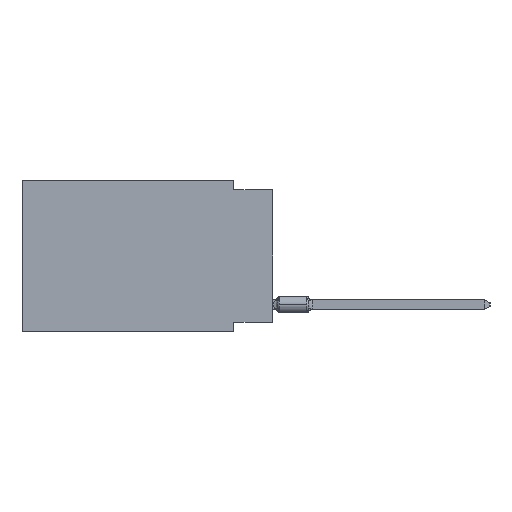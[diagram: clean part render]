
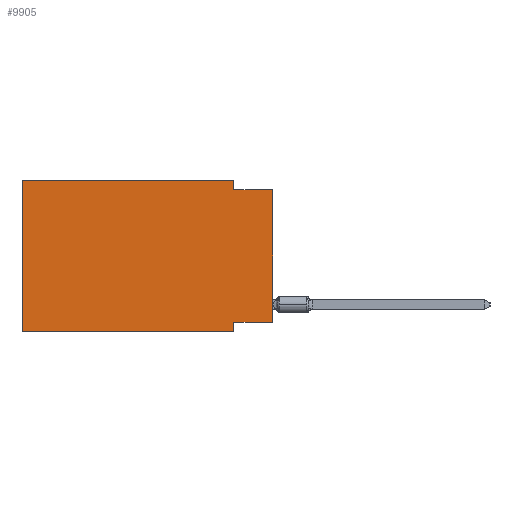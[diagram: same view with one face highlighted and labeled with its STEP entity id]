
A CAD part, left-side view. The second image highlights one B-rep face of the part: STEP entity #9905.
In plain terms, the highlighted planar face has unit normal (-1, 0, 0).
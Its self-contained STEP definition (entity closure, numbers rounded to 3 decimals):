
#143 = CARTESIAN_POINT ( 'NONE',  ( 0., 2.54, 0. ) ) ;
#326 = VERTEX_POINT ( 'NONE', #11461 ) ;
#494 = FACE_OUTER_BOUND ( 'NONE', #1102, .T. ) ;
#961 = CARTESIAN_POINT ( 'NONE',  ( 0., 0., -0.635 ) ) ;
#1102 = EDGE_LOOP ( 'NONE', ( #20735, #1895, #9198, #14807, #5593, #32313, #19526, #20743 ) ) ;
#1895 = ORIENTED_EDGE ( 'NONE', *, *, #18748, .F. ) ;
#3197 = CARTESIAN_POINT ( 'NONE',  ( 0., 16.383, -9.906 ) ) ;
#3350 = CARTESIAN_POINT ( 'NONE',  ( 0., 2.54, -0.635 ) ) ;
#3831 = CARTESIAN_POINT ( 'NONE',  ( 0., 2.54, -9.906 ) ) ;
#4923 = VECTOR ( 'NONE', #26231, 1000. ) ;
#5193 = CARTESIAN_POINT ( 'NONE',  ( 0., 0., -9.271 ) ) ;
#5593 = ORIENTED_EDGE ( 'NONE', *, *, #16250, .F. ) ;
#5747 = VERTEX_POINT ( 'NONE', #3831 ) ;
#6267 = VECTOR ( 'NONE', #8050, 1000. ) ;
#6835 = CARTESIAN_POINT ( 'NONE',  ( 0., 16.383, 0. ) ) ;
#7115 = VECTOR ( 'NONE', #19838, 1000. ) ;
#7275 = CARTESIAN_POINT ( 'NONE',  ( 0., 0., 0. ) ) ;
#8050 = DIRECTION ( 'NONE',  ( 0., 0., -1. ) ) ;
#8381 = VERTEX_POINT ( 'NONE', #3350 ) ;
#8400 = DIRECTION ( 'NONE',  ( 1., 0., 0. ) ) ;
#8706 = VERTEX_POINT ( 'NONE', #24206 ) ;
#9198 = ORIENTED_EDGE ( 'NONE', *, *, #11082, .F. ) ;
#9905 = ADVANCED_FACE ( 'NONE', ( #494 ), #29441, .F. ) ;
#10985 = LINE ( 'NONE', #32408, #23893 ) ;
#10995 = VERTEX_POINT ( 'NONE', #20362 ) ;
#11050 = EDGE_CURVE ( 'NONE', #8706, #5747, #25978, .T. ) ;
#11082 = EDGE_CURVE ( 'NONE', #30233, #8381, #24207, .T. ) ;
#11192 = DIRECTION ( 'NONE',  ( 0., 0., -1. ) ) ;
#11461 = CARTESIAN_POINT ( 'NONE',  ( 0., 0., -9.271 ) ) ;
#11488 = EDGE_CURVE ( 'NONE', #326, #8706, #26615, .T. ) ;
#12024 = VERTEX_POINT ( 'NONE', #961 ) ;
#12416 = AXIS2_PLACEMENT_3D ( 'NONE', #18935, #8400, #11192 ) ;
#13024 = LINE ( 'NONE', #26041, #29037 ) ;
#13339 = VECTOR ( 'NONE', #21461, 1000. ) ;
#14593 = VERTEX_POINT ( 'NONE', #18699 ) ;
#14807 = ORIENTED_EDGE ( 'NONE', *, *, #17193, .F. ) ;
#16250 = EDGE_CURVE ( 'NONE', #10995, #14593, #10985, .T. ) ;
#17193 = EDGE_CURVE ( 'NONE', #14593, #30233, #27909, .T. ) ;
#18699 = CARTESIAN_POINT ( 'NONE',  ( 0., 16.383, 0. ) ) ;
#18748 = EDGE_CURVE ( 'NONE', #8381, #12024, #13024, .T. ) ;
#18935 = CARTESIAN_POINT ( 'NONE',  ( 0., 16.383, 0. ) ) ;
#19059 = DIRECTION ( 'NONE',  ( 0., 1., 0. ) ) ;
#19269 = DIRECTION ( 'NONE',  ( 0., 0., 1. ) ) ;
#19526 = ORIENTED_EDGE ( 'NONE', *, *, #11050, .F. ) ;
#19595 = EDGE_CURVE ( 'NONE', #10995, #5747, #34612, .T. ) ;
#19838 = DIRECTION ( 'NONE',  ( 0., -1., 0. ) ) ;
#20362 = CARTESIAN_POINT ( 'NONE',  ( 0., 16.383, -9.906 ) ) ;
#20735 = ORIENTED_EDGE ( 'NONE', *, *, #27007, .T. ) ;
#20743 = ORIENTED_EDGE ( 'NONE', *, *, #11488, .F. ) ;
#21248 = CARTESIAN_POINT ( 'NONE',  ( 0., 2.54, 0. ) ) ;
#21288 = DIRECTION ( 'NONE',  ( 0., -1., 0. ) ) ;
#21399 = VECTOR ( 'NONE', #19059, 1000. ) ;
#21461 = DIRECTION ( 'NONE',  ( 0., -1., 0. ) ) ;
#23893 = VECTOR ( 'NONE', #19269, 1000. ) ;
#24206 = CARTESIAN_POINT ( 'NONE',  ( 0., 2.54, -9.271 ) ) ;
#24207 = LINE ( 'NONE', #143, #27656 ) ;
#25978 = LINE ( 'NONE', #32604, #6267 ) ;
#26041 = CARTESIAN_POINT ( 'NONE',  ( 0., 0., -0.635 ) ) ;
#26231 = DIRECTION ( 'NONE',  ( 0., 0., 1. ) ) ;
#26615 = LINE ( 'NONE', #5193, #21399 ) ;
#26653 = DIRECTION ( 'NONE',  ( 0., 0., -1. ) ) ;
#27007 = EDGE_CURVE ( 'NONE', #326, #12024, #28848, .T. ) ;
#27656 = VECTOR ( 'NONE', #26653, 1000. ) ;
#27909 = LINE ( 'NONE', #6835, #7115 ) ;
#28848 = LINE ( 'NONE', #7275, #4923 ) ;
#29037 = VECTOR ( 'NONE', #21288, 1000. ) ;
#29441 = PLANE ( 'NONE',  #12416 ) ;
#30233 = VERTEX_POINT ( 'NONE', #21248 ) ;
#32313 = ORIENTED_EDGE ( 'NONE', *, *, #19595, .T. ) ;
#32408 = CARTESIAN_POINT ( 'NONE',  ( 0., 16.383, 0. ) ) ;
#32604 = CARTESIAN_POINT ( 'NONE',  ( 0., 2.54, -9.906 ) ) ;
#34612 = LINE ( 'NONE', #3197, #13339 ) ;
